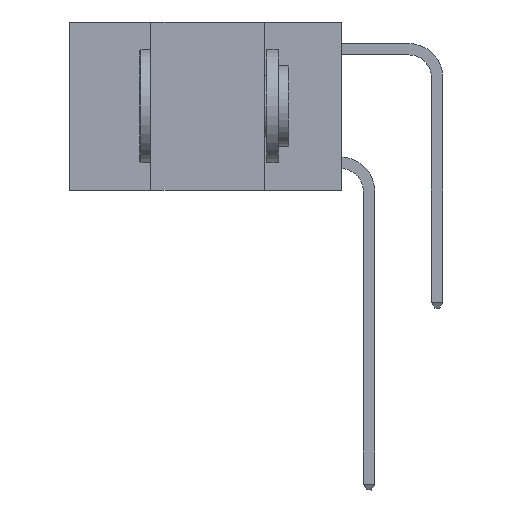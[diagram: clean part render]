
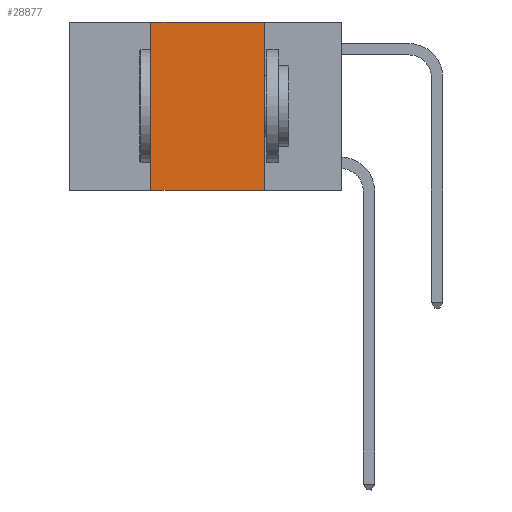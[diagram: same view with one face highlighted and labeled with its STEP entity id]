
A CAD part, left-side view. The second image highlights one B-rep face of the part: STEP entity #28877.
In plain terms, the highlighted planar face has unit normal (-1, 0, 0).
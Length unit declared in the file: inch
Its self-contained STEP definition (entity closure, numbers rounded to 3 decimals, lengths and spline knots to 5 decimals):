
#249 = EDGE_CURVE ( 'NONE', #6828, #12220, #29025, .T. ) ;
#688 = ORIENTED_EDGE ( 'NONE', *, *, #13310, .F. ) ;
#945 = VECTOR ( 'NONE', #7701, 39.37008 ) ;
#998 = CARTESIAN_POINT ( 'NONE',  ( 0., 0.17, 0. ) ) ;
#1044 = ORIENTED_EDGE ( 'NONE', *, *, #249, .F. ) ;
#3028 = AXIS2_PLACEMENT_3D ( 'NONE', #9529, #11957, #28377 ) ;
#4361 = VECTOR ( 'NONE', #15528, 39.37008 ) ;
#5268 = EDGE_LOOP ( 'NONE', ( #1044, #688, #9548, #24331 ) ) ;
#5722 = VERTEX_POINT ( 'NONE', #18106 ) ;
#5995 = CARTESIAN_POINT ( 'NONE',  ( 0., 0.17, -0.37 ) ) ;
#6828 = VERTEX_POINT ( 'NONE', #998 ) ;
#7164 = PLANE ( 'NONE',  #3028 ) ;
#7701 = DIRECTION ( 'NONE',  ( 0., -1., 0. ) ) ;
#9529 = CARTESIAN_POINT ( 'NONE',  ( 0., 0.6, 0. ) ) ;
#9548 = ORIENTED_EDGE ( 'NONE', *, *, #12487, .F. ) ;
#10096 = CARTESIAN_POINT ( 'NONE',  ( 0., 0.6, 0. ) ) ;
#10641 = LINE ( 'NONE', #13158, #4361 ) ;
#11957 = DIRECTION ( 'NONE',  ( 1., 0., 0. ) ) ;
#12171 = CARTESIAN_POINT ( 'NONE',  ( 0., 0.17, 0. ) ) ;
#12220 = VERTEX_POINT ( 'NONE', #5995 ) ;
#12487 = EDGE_CURVE ( 'NONE', #13850, #5722, #28891, .T. ) ;
#13158 = CARTESIAN_POINT ( 'NONE',  ( 0., 0.6, -0.37 ) ) ;
#13310 = EDGE_CURVE ( 'NONE', #5722, #6828, #26780, .T. ) ;
#13850 = VERTEX_POINT ( 'NONE', #16686 ) ;
#15528 = DIRECTION ( 'NONE',  ( 0., -1., 0. ) ) ;
#16686 = CARTESIAN_POINT ( 'NONE',  ( 0., 0.42, -0.37 ) ) ;
#17883 = VECTOR ( 'NONE', #25787, 39.37008 ) ;
#18106 = CARTESIAN_POINT ( 'NONE',  ( 0., 0.42, 0. ) ) ;
#21740 = EDGE_CURVE ( 'NONE', #13850, #12220, #10641, .T. ) ;
#22485 = FACE_OUTER_BOUND ( 'NONE', #5268, .T. ) ;
#23451 = CARTESIAN_POINT ( 'NONE',  ( 0., 0.42, 0. ) ) ;
#24331 = ORIENTED_EDGE ( 'NONE', *, *, #21740, .T. ) ;
#24647 = DIRECTION ( 'NONE',  ( 0., 0., -1. ) ) ;
#25787 = DIRECTION ( 'NONE',  ( 0., 0., 1. ) ) ;
#26780 = LINE ( 'NONE', #10096, #945 ) ;
#28289 = VECTOR ( 'NONE', #24647, 39.37008 ) ;
#28377 = DIRECTION ( 'NONE',  ( 0., 0., -1. ) ) ;
#28877 = ADVANCED_FACE ( 'NONE', ( #22485 ), #7164, .F. ) ;
#28891 = LINE ( 'NONE', #23451, #17883 ) ;
#29025 = LINE ( 'NONE', #12171, #28289 ) ;
